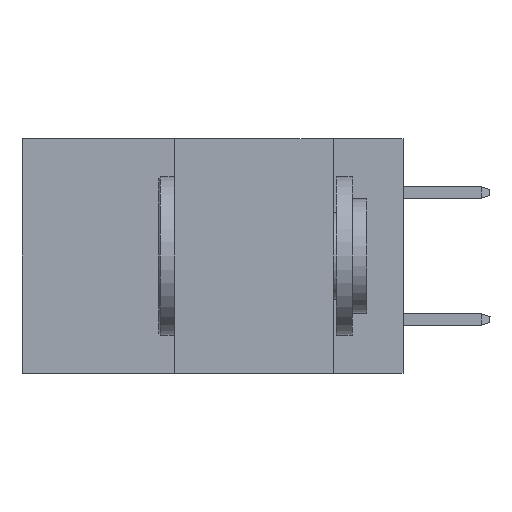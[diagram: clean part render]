
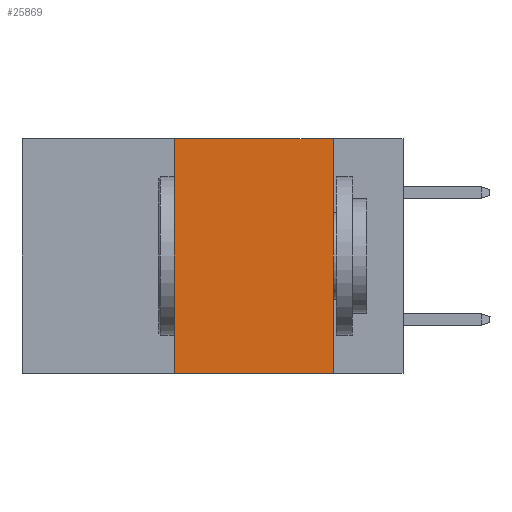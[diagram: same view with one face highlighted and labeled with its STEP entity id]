
A CAD part, left-side view. The second image highlights one B-rep face of the part: STEP entity #25869.
In plain terms, the highlighted planar face has unit normal (-1, 0, 0).
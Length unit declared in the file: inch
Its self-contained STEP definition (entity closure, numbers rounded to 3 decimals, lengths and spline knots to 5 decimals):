
#1661 = DIRECTION ( 'NONE',  ( 0., -1., 0. ) ) ;
#1683 = CARTESIAN_POINT ( 'NONE',  ( 0., 0.36, 0. ) ) ;
#2532 = AXIS2_PLACEMENT_3D ( 'NONE', #9670, #24039, #9798 ) ;
#2806 = EDGE_LOOP ( 'NONE', ( #21335, #5515, #3486, #6948 ) ) ;
#3446 = VERTEX_POINT ( 'NONE', #1683 ) ;
#3486 = ORIENTED_EDGE ( 'NONE', *, *, #17509, .F. ) ;
#4357 = CARTESIAN_POINT ( 'NONE',  ( 0., 0.36, -0.37 ) ) ;
#4360 = VECTOR ( 'NONE', #15422, 39.37008 ) ;
#5515 = ORIENTED_EDGE ( 'NONE', *, *, #23234, .F. ) ;
#6893 = VERTEX_POINT ( 'NONE', #4357 ) ;
#6948 = ORIENTED_EDGE ( 'NONE', *, *, #18854, .T. ) ;
#7192 = DIRECTION ( 'NONE',  ( 0., -1., 0. ) ) ;
#7319 = LINE ( 'NONE', #19363, #24157 ) ;
#7876 = VERTEX_POINT ( 'NONE', #8199 ) ;
#8199 = CARTESIAN_POINT ( 'NONE',  ( 0., 0.11, 0. ) ) ;
#8397 = VECTOR ( 'NONE', #21341, 39.37008 ) ;
#9233 = EDGE_CURVE ( 'NONE', #7876, #18094, #21840, .T. ) ;
#9670 = CARTESIAN_POINT ( 'NONE',  ( 0., 0.6, 0. ) ) ;
#9798 = DIRECTION ( 'NONE',  ( 0., 0., -1. ) ) ;
#10808 = VECTOR ( 'NONE', #1661, 39.37008 ) ;
#11642 = CARTESIAN_POINT ( 'NONE',  ( 0., 0.6, 0. ) ) ;
#13438 = LINE ( 'NONE', #17158, #4360 ) ;
#15422 = DIRECTION ( 'NONE',  ( 0., 0., 1. ) ) ;
#15624 = PLANE ( 'NONE',  #2532 ) ;
#17158 = CARTESIAN_POINT ( 'NONE',  ( 0., 0.36, 0. ) ) ;
#17455 = LINE ( 'NONE', #11642, #10808 ) ;
#17509 = EDGE_CURVE ( 'NONE', #6893, #3446, #13438, .T. ) ;
#18094 = VERTEX_POINT ( 'NONE', #21768 ) ;
#18854 = EDGE_CURVE ( 'NONE', #6893, #18094, #7319, .T. ) ;
#19363 = CARTESIAN_POINT ( 'NONE',  ( 0., 0.6, -0.37 ) ) ;
#21335 = ORIENTED_EDGE ( 'NONE', *, *, #9233, .F. ) ;
#21341 = DIRECTION ( 'NONE',  ( 0., 0., -1. ) ) ;
#21768 = CARTESIAN_POINT ( 'NONE',  ( 0., 0.11, -0.37 ) ) ;
#21840 = LINE ( 'NONE', #23411, #8397 ) ;
#21944 = FACE_OUTER_BOUND ( 'NONE', #2806, .T. ) ;
#23234 = EDGE_CURVE ( 'NONE', #3446, #7876, #17455, .T. ) ;
#23411 = CARTESIAN_POINT ( 'NONE',  ( 0., 0.11, 0. ) ) ;
#24039 = DIRECTION ( 'NONE',  ( 1., 0., 0. ) ) ;
#24157 = VECTOR ( 'NONE', #7192, 39.37008 ) ;
#25869 = ADVANCED_FACE ( 'NONE', ( #21944 ), #15624, .F. ) ;
